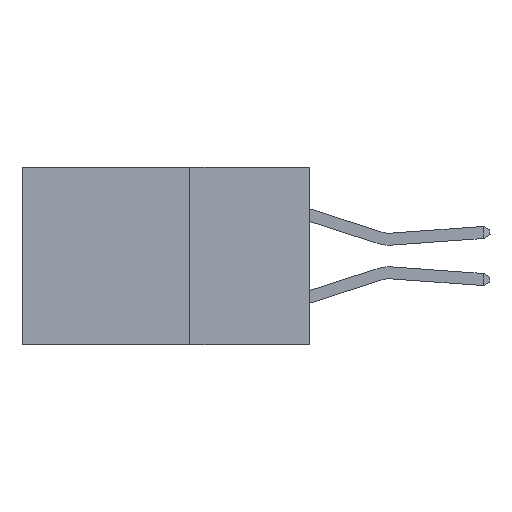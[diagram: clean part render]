
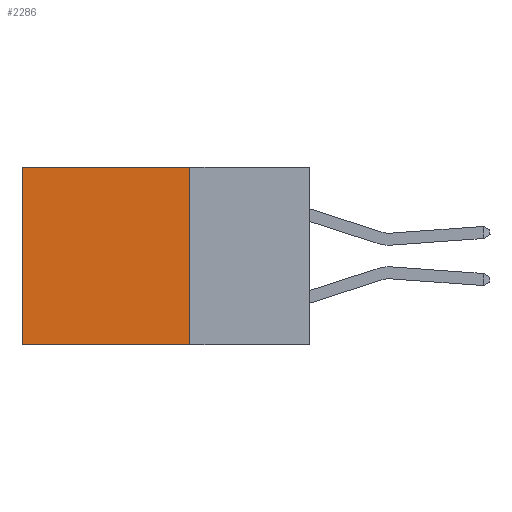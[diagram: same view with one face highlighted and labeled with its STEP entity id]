
A CAD part, left-side view. The second image highlights one B-rep face of the part: STEP entity #2286.
In plain terms, the highlighted planar face has unit normal (-1, 0, 0).
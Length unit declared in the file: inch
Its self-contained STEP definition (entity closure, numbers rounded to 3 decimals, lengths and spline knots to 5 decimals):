
#1203 = VECTOR ( 'NONE', #3668, 39.37008 ) ;
#1652 = VECTOR ( 'NONE', #12688, 39.37008 ) ;
#1710 = VECTOR ( 'NONE', #3997, 39.37008 ) ;
#2051 = VERTEX_POINT ( 'NONE', #8591 ) ;
#2286 = ADVANCED_FACE ( 'NONE', ( #10177 ), #11289, .F. ) ;
#2502 = LINE ( 'NONE', #6996, #1203 ) ;
#2635 = CARTESIAN_POINT ( 'NONE',  ( 0.2615, 0.25, -0.37 ) ) ;
#3131 = CARTESIAN_POINT ( 'NONE',  ( 0.2615, 0.25, 0. ) ) ;
#3668 = DIRECTION ( 'NONE',  ( 0., 1., 0. ) ) ;
#3928 = CARTESIAN_POINT ( 'NONE',  ( 0.2615, 0.6, -0.37 ) ) ;
#3997 = DIRECTION ( 'NONE',  ( 0., 1., 0. ) ) ;
#4237 = VERTEX_POINT ( 'NONE', #3131 ) ;
#4619 = CARTESIAN_POINT ( 'NONE',  ( 0.2615, 0.25, -0.37 ) ) ;
#4790 = ORIENTED_EDGE ( 'NONE', *, *, #11533, .F. ) ;
#5043 = ORIENTED_EDGE ( 'NONE', *, *, #6065, .T. ) ;
#5468 = CARTESIAN_POINT ( 'NONE',  ( 0.2615, 0.6, 0. ) ) ;
#5998 = EDGE_CURVE ( 'NONE', #4237, #12232, #9271, .T. ) ;
#6034 = LINE ( 'NONE', #3928, #10990 ) ;
#6065 = EDGE_CURVE ( 'NONE', #12232, #12115, #6034, .T. ) ;
#6558 = ORIENTED_EDGE ( 'NONE', *, *, #5998, .T. ) ;
#6996 = CARTESIAN_POINT ( 'NONE',  ( 0.2615, 0.25, -0.37 ) ) ;
#8176 = DIRECTION ( 'NONE',  ( 0., 0., -1. ) ) ;
#8591 = CARTESIAN_POINT ( 'NONE',  ( 0.2615, 0.25, -0.37 ) ) ;
#9271 = LINE ( 'NONE', #13875, #1710 ) ;
#10158 = AXIS2_PLACEMENT_3D ( 'NONE', #4619, #13355, #11212 ) ;
#10177 = FACE_OUTER_BOUND ( 'NONE', #11366, .T. ) ;
#10418 = EDGE_CURVE ( 'NONE', #4237, #2051, #10624, .T. ) ;
#10624 = LINE ( 'NONE', #2635, #1652 ) ;
#10990 = VECTOR ( 'NONE', #8176, 39.37008 ) ;
#11212 = DIRECTION ( 'NONE',  ( 0., 0., -1. ) ) ;
#11289 = PLANE ( 'NONE',  #10158 ) ;
#11366 = EDGE_LOOP ( 'NONE', ( #5043, #4790, #12896, #6558 ) ) ;
#11533 = EDGE_CURVE ( 'NONE', #2051, #12115, #2502, .T. ) ;
#12115 = VERTEX_POINT ( 'NONE', #13611 ) ;
#12232 = VERTEX_POINT ( 'NONE', #5468 ) ;
#12688 = DIRECTION ( 'NONE',  ( 0., 0., -1. ) ) ;
#12896 = ORIENTED_EDGE ( 'NONE', *, *, #10418, .F. ) ;
#13355 = DIRECTION ( 'NONE',  ( 1., 0., 0. ) ) ;
#13611 = CARTESIAN_POINT ( 'NONE',  ( 0.2615, 0.6, -0.37 ) ) ;
#13875 = CARTESIAN_POINT ( 'NONE',  ( 0.2615, 0.25, 0. ) ) ;
